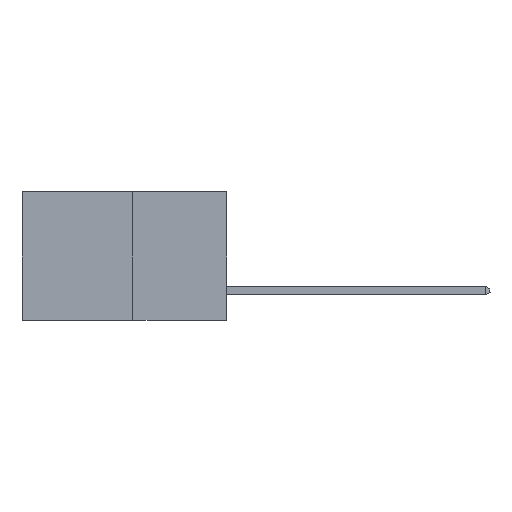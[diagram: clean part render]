
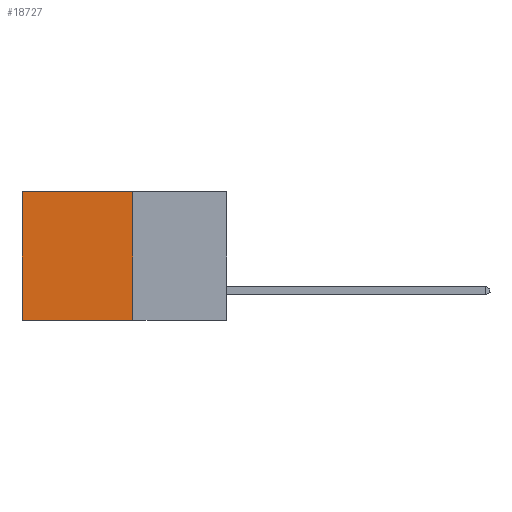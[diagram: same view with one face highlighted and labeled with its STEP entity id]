
A CAD part, left-side view. The second image highlights one B-rep face of the part: STEP entity #18727.
In plain terms, the highlighted planar face has unit normal (-1, 0, 0).
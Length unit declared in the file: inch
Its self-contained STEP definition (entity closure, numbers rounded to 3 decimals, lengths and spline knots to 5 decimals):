
#1784 = FACE_OUTER_BOUND ( 'NONE', #17351, .T. ) ;
#1875 = DIRECTION ( 'NONE',  ( 0., 1., 0. ) ) ;
#2301 = CARTESIAN_POINT ( 'NONE',  ( 0.277, 0.27, -0.37 ) ) ;
#3017 = CARTESIAN_POINT ( 'NONE',  ( 0.277, 0.59, -0.37 ) ) ;
#3023 = PLANE ( 'NONE',  #10746 ) ;
#3806 = ORIENTED_EDGE ( 'NONE', *, *, #7795, .T. ) ;
#4379 = DIRECTION ( 'NONE',  ( 0., 0., -1. ) ) ;
#5173 = DIRECTION ( 'NONE',  ( 0., 0., -1. ) ) ;
#6121 = CARTESIAN_POINT ( 'NONE',  ( 0.277, 0.27, 0. ) ) ;
#6127 = EDGE_CURVE ( 'NONE', #6153, #26467, #27454, .T. ) ;
#6153 = VERTEX_POINT ( 'NONE', #11688 ) ;
#6905 = CARTESIAN_POINT ( 'NONE',  ( 0.277, 0.59, -0.37 ) ) ;
#6964 = VERTEX_POINT ( 'NONE', #27069 ) ;
#7747 = ORIENTED_EDGE ( 'NONE', *, *, #6127, .T. ) ;
#7795 = EDGE_CURVE ( 'NONE', #6964, #6153, #18115, .T. ) ;
#8294 = DIRECTION ( 'NONE',  ( 0., 1., 0. ) ) ;
#8400 = EDGE_CURVE ( 'NONE', #6964, #17004, #25383, .T. ) ;
#10386 = VECTOR ( 'NONE', #20327, 39.37008 ) ;
#10746 = AXIS2_PLACEMENT_3D ( 'NONE', #24405, #18166, #5173 ) ;
#11262 = VECTOR ( 'NONE', #1875, 39.37008 ) ;
#11688 = CARTESIAN_POINT ( 'NONE',  ( 0.277, 0.59, 0. ) ) ;
#12640 = CARTESIAN_POINT ( 'NONE',  ( 0.277, 0.27, -0.37 ) ) ;
#16346 = CARTESIAN_POINT ( 'NONE',  ( 0.277, 0.27, -0.37 ) ) ;
#16700 = ORIENTED_EDGE ( 'NONE', *, *, #27567, .F. ) ;
#17004 = VERTEX_POINT ( 'NONE', #16346 ) ;
#17068 = ORIENTED_EDGE ( 'NONE', *, *, #8400, .F. ) ;
#17351 = EDGE_LOOP ( 'NONE', ( #7747, #16700, #17068, #3806 ) ) ;
#18115 = LINE ( 'NONE', #6121, #18803 ) ;
#18166 = DIRECTION ( 'NONE',  ( 1., 0., 0. ) ) ;
#18727 = ADVANCED_FACE ( 'NONE', ( #1784 ), #3023, .F. ) ;
#18803 = VECTOR ( 'NONE', #8294, 39.37008 ) ;
#20327 = DIRECTION ( 'NONE',  ( 0., 0., -1. ) ) ;
#22755 = LINE ( 'NONE', #12640, #11262 ) ;
#24405 = CARTESIAN_POINT ( 'NONE',  ( 0.277, 0.27, -0.37 ) ) ;
#24730 = VECTOR ( 'NONE', #4379, 39.37008 ) ;
#25383 = LINE ( 'NONE', #2301, #24730 ) ;
#26467 = VERTEX_POINT ( 'NONE', #6905 ) ;
#27069 = CARTESIAN_POINT ( 'NONE',  ( 0.277, 0.27, 0. ) ) ;
#27454 = LINE ( 'NONE', #3017, #10386 ) ;
#27567 = EDGE_CURVE ( 'NONE', #17004, #26467, #22755, .T. ) ;
